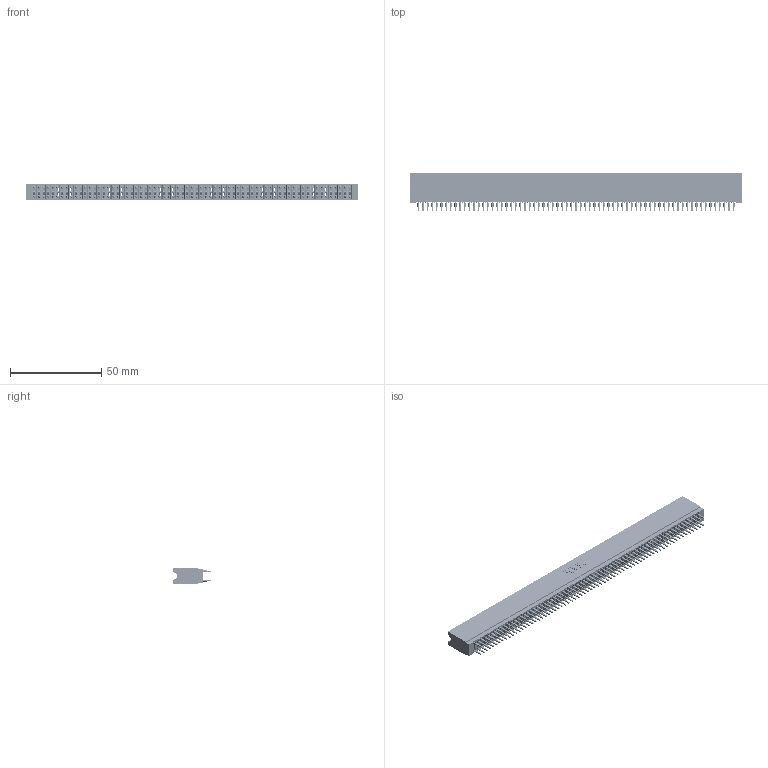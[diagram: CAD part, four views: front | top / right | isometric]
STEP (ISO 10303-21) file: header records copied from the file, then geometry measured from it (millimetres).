
FILE_DESCRIPTION (( 'STEP AP203' ), '1' );
FILE_NAME ('745-138-560-206.STEP', '2026-02-27T03:37:52', ( '' ), ( '' ), 'SwSTEP 2.0', 'SolidWorks 2023', '' );
FILE_SCHEMA (( 'CONFIG_CONTROL_DESIGN' ));
Length unit declared in the file: millimetre
Products named in the file (3): 745-138-560-206; 745-292-001_560; 745 Part_Insulator Option - 06
Assembly tree (139 placements, depth 2):
  745-138-560-206
    745 Part_Insulator Option - 06
    745-292-001_560  x138
Bounding box: 181.86 x 21.22 x 8.89 mm (x, y, z)
Volume: 16702.9 mm3; surface area: 36784.9 mm2
Topology: 139 solids, 139 shells, 13689 faces, 37451 edges, 23770 vertices
Faces by surface type: plane 7094, cylinder 3007, bspline 2760, torus 828
Entity records: 112820 total; most frequent: CARTESIAN_POINT 20064, ORIENTED_EDGE 19554, DIRECTION 17063, EDGE_CURVE 9777, VECTOR 9173, LINE 9173, VERTEX_POINT 6234, AXIS2_PLACEMENT_3D 3945
